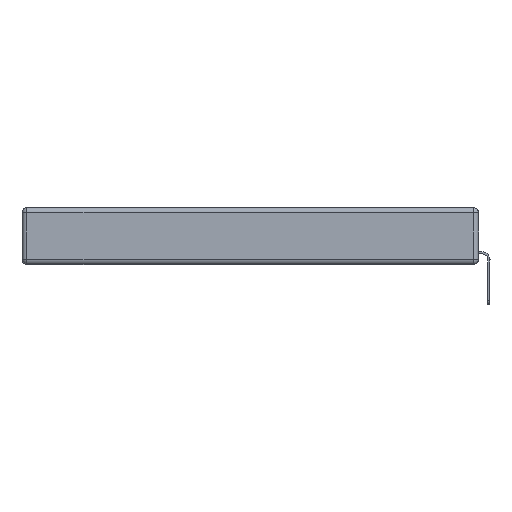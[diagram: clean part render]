
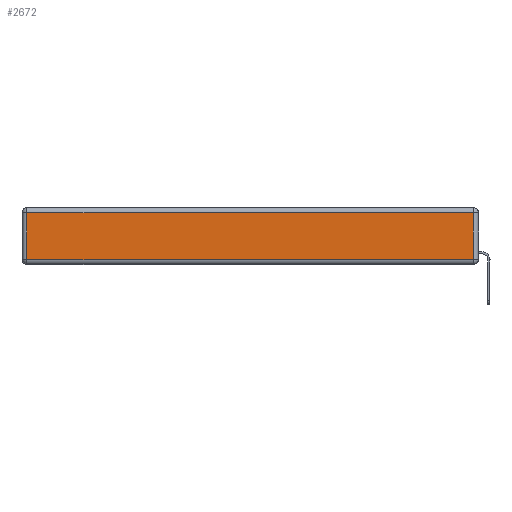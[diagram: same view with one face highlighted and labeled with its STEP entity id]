
A CAD part, left-side view. The second image highlights one B-rep face of the part: STEP entity #2672.
In plain terms, the highlighted planar face has unit normal (-1, 0, 0).
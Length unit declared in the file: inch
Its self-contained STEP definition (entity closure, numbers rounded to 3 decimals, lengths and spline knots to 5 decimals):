
#559 = CARTESIAN_POINT ( 'NONE',  ( 0., 2.72, -0.343 ) ) ;
#861 = EDGE_LOOP ( 'NONE', ( #14166, #12800, #14487, #11083 ) ) ;
#1003 = CARTESIAN_POINT ( 'NONE',  ( 0., 2.72, -0.03 ) ) ;
#1379 = DIRECTION ( 'NONE',  ( 0., -1., 0. ) ) ;
#1504 = DIRECTION ( 'NONE',  ( 0., 0., -1. ) ) ;
#2494 = PLANE ( 'NONE',  #12298 ) ;
#2672 = ADVANCED_FACE ( 'NONE', ( #8353 ), #2494, .T. ) ;
#3552 = EDGE_CURVE ( 'NONE', #9046, #5346, #6414, .T. ) ;
#3707 = EDGE_CURVE ( 'NONE', #8011, #7940, #9052, .T. ) ;
#4387 = CARTESIAN_POINT ( 'NONE',  ( 0., 0.03, -0.343 ) ) ;
#4840 = DIRECTION ( 'NONE',  ( 0., 0., 1. ) ) ;
#5346 = VERTEX_POINT ( 'NONE', #5684 ) ;
#5684 = CARTESIAN_POINT ( 'NONE',  ( 0., 2.72, -0.313 ) ) ;
#5724 = EDGE_CURVE ( 'NONE', #7940, #9046, #13618, .T. ) ;
#6414 = LINE ( 'NONE', #559, #12880 ) ;
#6749 = CARTESIAN_POINT ( 'NONE',  ( 0., 2.75, -0.03 ) ) ;
#7029 = VECTOR ( 'NONE', #1379, 39.37008 ) ;
#7240 = DIRECTION ( 'NONE',  ( -1., 0., 0. ) ) ;
#7600 = CARTESIAN_POINT ( 'NONE',  ( 0., 0.03, -0.313 ) ) ;
#7869 = EDGE_CURVE ( 'NONE', #5346, #8011, #9716, .T. ) ;
#7940 = VERTEX_POINT ( 'NONE', #10820 ) ;
#8011 = VERTEX_POINT ( 'NONE', #7600 ) ;
#8353 = FACE_OUTER_BOUND ( 'NONE', #861, .T. ) ;
#9046 = VERTEX_POINT ( 'NONE', #1003 ) ;
#9052 = LINE ( 'NONE', #4387, #10359 ) ;
#9055 = VECTOR ( 'NONE', #15092, 39.37008 ) ;
#9676 = CARTESIAN_POINT ( 'NONE',  ( 0., 0., -0.343 ) ) ;
#9716 = LINE ( 'NONE', #14453, #7029 ) ;
#10359 = VECTOR ( 'NONE', #14817, 39.37008 ) ;
#10820 = CARTESIAN_POINT ( 'NONE',  ( 0., 0.03, -0.03 ) ) ;
#11083 = ORIENTED_EDGE ( 'NONE', *, *, #3552, .T. ) ;
#12298 = AXIS2_PLACEMENT_3D ( 'NONE', #9676, #7240, #4840 ) ;
#12800 = ORIENTED_EDGE ( 'NONE', *, *, #3707, .T. ) ;
#12880 = VECTOR ( 'NONE', #1504, 39.37008 ) ;
#13618 = LINE ( 'NONE', #6749, #9055 ) ;
#14166 = ORIENTED_EDGE ( 'NONE', *, *, #7869, .T. ) ;
#14453 = CARTESIAN_POINT ( 'NONE',  ( 0., 0., -0.313 ) ) ;
#14487 = ORIENTED_EDGE ( 'NONE', *, *, #5724, .T. ) ;
#14817 = DIRECTION ( 'NONE',  ( 0., 0., 1. ) ) ;
#15092 = DIRECTION ( 'NONE',  ( 0., 1., 0. ) ) ;
